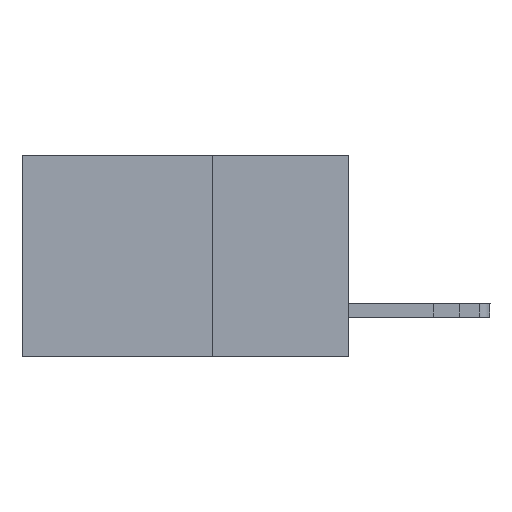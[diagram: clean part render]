
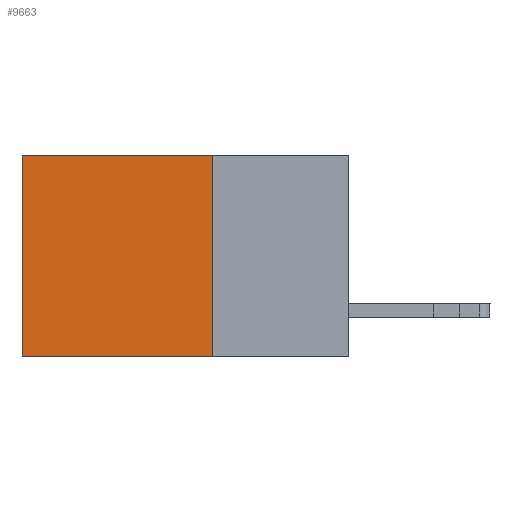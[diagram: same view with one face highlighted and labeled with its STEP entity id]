
A CAD part, left-side view. The second image highlights one B-rep face of the part: STEP entity #9663.
In plain terms, the highlighted planar face has unit normal (-1, 0, 0).
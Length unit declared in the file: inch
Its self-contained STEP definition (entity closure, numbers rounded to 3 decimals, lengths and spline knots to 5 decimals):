
#279 = CARTESIAN_POINT ( 'NONE',  ( 0.298, 0.25, 0. ) ) ;
#631 = ORIENTED_EDGE ( 'NONE', *, *, #2102, .F. ) ;
#1873 = CARTESIAN_POINT ( 'NONE',  ( 0.298, 0.25, 0. ) ) ;
#2102 = EDGE_CURVE ( 'NONE', #16768, #18403, #3403, .T. ) ;
#2236 = CARTESIAN_POINT ( 'NONE',  ( 0.298, 0.25, -0.37 ) ) ;
#3403 = LINE ( 'NONE', #4819, #10390 ) ;
#3899 = EDGE_LOOP ( 'NONE', ( #5449, #631, #9372, #5733 ) ) ;
#4053 = DIRECTION ( 'NONE',  ( 0., 1., 0. ) ) ;
#4560 = EDGE_CURVE ( 'NONE', #13067, #16768, #15882, .T. ) ;
#4819 = CARTESIAN_POINT ( 'NONE',  ( 0.298, 0.25, -0.37 ) ) ;
#5152 = CARTESIAN_POINT ( 'NONE',  ( 0.298, 0.6, 0. ) ) ;
#5203 = EDGE_CURVE ( 'NONE', #13067, #14420, #19479, .T. ) ;
#5344 = CARTESIAN_POINT ( 'NONE',  ( 0.298, 0.6, 0. ) ) ;
#5449 = ORIENTED_EDGE ( 'NONE', *, *, #13164, .T. ) ;
#5574 = CARTESIAN_POINT ( 'NONE',  ( 0.298, 0.25, 0. ) ) ;
#5733 = ORIENTED_EDGE ( 'NONE', *, *, #5203, .T. ) ;
#6968 = VECTOR ( 'NONE', #11108, 39.37008 ) ;
#7917 = VECTOR ( 'NONE', #11848, 39.37008 ) ;
#8173 = DIRECTION ( 'NONE',  ( 1., 0., 0. ) ) ;
#8266 = CARTESIAN_POINT ( 'NONE',  ( 0.298, 0.25, 0. ) ) ;
#9372 = ORIENTED_EDGE ( 'NONE', *, *, #4560, .F. ) ;
#9663 = ADVANCED_FACE ( 'NONE', ( #16178 ), #17400, .F. ) ;
#9696 = DIRECTION ( 'NONE',  ( 0., 0., -1. ) ) ;
#10390 = VECTOR ( 'NONE', #14265, 39.37008 ) ;
#11108 = DIRECTION ( 'NONE',  ( 0., 0., -1. ) ) ;
#11651 = LINE ( 'NONE', #5344, #7917 ) ;
#11848 = DIRECTION ( 'NONE',  ( 0., 0., -1. ) ) ;
#13067 = VERTEX_POINT ( 'NONE', #279 ) ;
#13164 = EDGE_CURVE ( 'NONE', #14420, #18403, #11651, .T. ) ;
#14265 = DIRECTION ( 'NONE',  ( 0., 1., 0. ) ) ;
#14420 = VERTEX_POINT ( 'NONE', #5152 ) ;
#14658 = VECTOR ( 'NONE', #4053, 39.37008 ) ;
#15882 = LINE ( 'NONE', #1873, #6968 ) ;
#16178 = FACE_OUTER_BOUND ( 'NONE', #3899, .T. ) ;
#16768 = VERTEX_POINT ( 'NONE', #2236 ) ;
#17400 = PLANE ( 'NONE',  #19446 ) ;
#18403 = VERTEX_POINT ( 'NONE', #19155 ) ;
#19155 = CARTESIAN_POINT ( 'NONE',  ( 0.298, 0.6, -0.37 ) ) ;
#19446 = AXIS2_PLACEMENT_3D ( 'NONE', #8266, #8173, #9696 ) ;
#19479 = LINE ( 'NONE', #5574, #14658 ) ;
